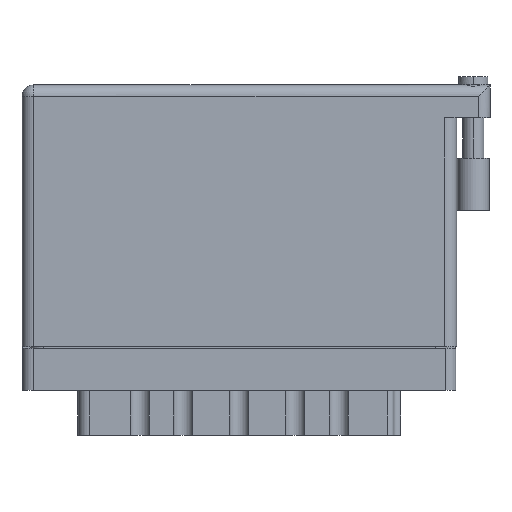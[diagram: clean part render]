
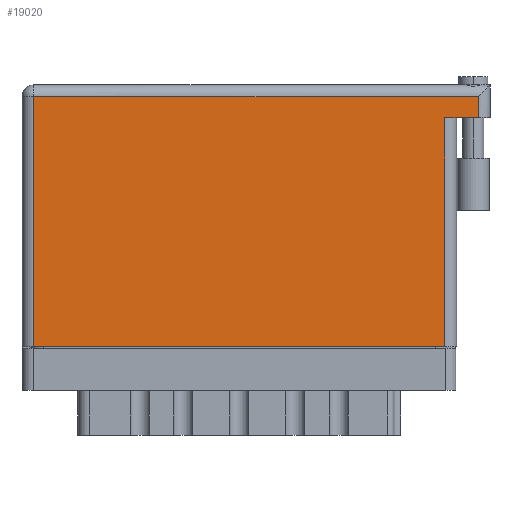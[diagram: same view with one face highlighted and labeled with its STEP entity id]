
A CAD part, front view. The second image highlights one B-rep face of the part: STEP entity #19020.
In plain terms, the highlighted face is planar.
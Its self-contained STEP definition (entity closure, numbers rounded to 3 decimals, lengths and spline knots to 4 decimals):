
#864 = CARTESIAN_POINT ( 'NONE',  ( 0.07, 1.496, 0. ) ) ;
#1656 = EDGE_CURVE ( 'NONE', #18155, #47281, #36971, .T. ) ;
#1996 = CARTESIAN_POINT ( 'NONE',  ( 0., 1.496, 0. ) ) ;
#2214 = LINE ( 'NONE', #2614, #45304 ) ;
#2614 = CARTESIAN_POINT ( 'NONE',  ( 0.07, 0., 0. ) ) ;
#2940 = EDGE_CURVE ( 'NONE', #47281, #40726, #33651, .T. ) ;
#4254 = EDGE_LOOP ( 'NONE', ( #26944, #7937, #6889, #48483, #14424, #35608 ) ) ;
#6889 = ORIENTED_EDGE ( 'NONE', *, *, #50073, .F. ) ;
#7937 = ORIENTED_EDGE ( 'NONE', *, *, #2940, .T. ) ;
#8254 = CARTESIAN_POINT ( 'NONE',  ( 2.73, 1.566, 0. ) ) ;
#11295 = VERTEX_POINT ( 'NONE', #34464 ) ;
#12789 = EDGE_CURVE ( 'NONE', #18784, #11295, #18122, .T. ) ;
#14424 = ORIENTED_EDGE ( 'NONE', *, *, #19552, .T. ) ;
#18122 = LINE ( 'NONE', #8254, #41901 ) ;
#18155 = VERTEX_POINT ( 'NONE', #53224 ) ;
#18784 = VERTEX_POINT ( 'NONE', #33214 ) ;
#19020 = ADVANCED_FACE ( 'NONE', ( #38254 ), #50979, .F. ) ;
#19140 = DIRECTION ( 'NONE',  ( 0., 0., -1. ) ) ;
#19277 = CARTESIAN_POINT ( 'NONE',  ( 2.53, 0., 0. ) ) ;
#19552 = EDGE_CURVE ( 'NONE', #11295, #43130, #40735, .T. ) ;
#26078 = DIRECTION ( 'NONE',  ( -1., 0., 0. ) ) ;
#26944 = ORIENTED_EDGE ( 'NONE', *, *, #1656, .T. ) ;
#27582 = DIRECTION ( 'NONE',  ( 0., -1., 0. ) ) ;
#28447 = AXIS2_PLACEMENT_3D ( 'NONE', #52037, #19140, #47901 ) ;
#28995 = CARTESIAN_POINT ( 'NONE',  ( 2.53, 1.369, 0. ) ) ;
#29802 = VECTOR ( 'NONE', #26078, 39.3701 ) ;
#31305 = DIRECTION ( 'NONE',  ( 1., 0., 0. ) ) ;
#32183 = EDGE_CURVE ( 'NONE', #43130, #18155, #2214, .T. ) ;
#32775 = LINE ( 'NONE', #42728, #50779 ) ;
#33046 = DIRECTION ( 'NONE',  ( 0., 1., 0. ) ) ;
#33214 = CARTESIAN_POINT ( 'NONE',  ( 2.73, 1.369, 0. ) ) ;
#33651 = LINE ( 'NONE', #28995, #34270 ) ;
#34270 = VECTOR ( 'NONE', #41038, 39.3701 ) ;
#34464 = CARTESIAN_POINT ( 'NONE',  ( 2.73, 1.496, 0. ) ) ;
#35129 = CARTESIAN_POINT ( 'NONE',  ( 0., 0., 0. ) ) ;
#35608 = ORIENTED_EDGE ( 'NONE', *, *, #32183, .T. ) ;
#36971 = LINE ( 'NONE', #35129, #38232 ) ;
#38232 = VECTOR ( 'NONE', #31305, 39.3701 ) ;
#38254 = FACE_OUTER_BOUND ( 'NONE', #4254, .T. ) ;
#40726 = VERTEX_POINT ( 'NONE', #49871 ) ;
#40735 = LINE ( 'NONE', #1996, #29802 ) ;
#41038 = DIRECTION ( 'NONE',  ( 0., 1., 0. ) ) ;
#41901 = VECTOR ( 'NONE', #33046, 39.3701 ) ;
#42728 = CARTESIAN_POINT ( 'NONE',  ( 2.8, 1.369, 0. ) ) ;
#43130 = VERTEX_POINT ( 'NONE', #864 ) ;
#45304 = VECTOR ( 'NONE', #27582, 39.3701 ) ;
#46872 = DIRECTION ( 'NONE',  ( -1., 0., 0. ) ) ;
#47281 = VERTEX_POINT ( 'NONE', #19277 ) ;
#47901 = DIRECTION ( 'NONE',  ( -1., 0., 0. ) ) ;
#48483 = ORIENTED_EDGE ( 'NONE', *, *, #12789, .T. ) ;
#49871 = CARTESIAN_POINT ( 'NONE',  ( 2.53, 1.369, 0. ) ) ;
#50073 = EDGE_CURVE ( 'NONE', #18784, #40726, #32775, .T. ) ;
#50779 = VECTOR ( 'NONE', #46872, 39.3701 ) ;
#50979 = PLANE ( 'NONE',  #28447 ) ;
#52037 = CARTESIAN_POINT ( 'NONE',  ( 0., 1.566, 0. ) ) ;
#53224 = CARTESIAN_POINT ( 'NONE',  ( 0.07, 0., 0. ) ) ;
